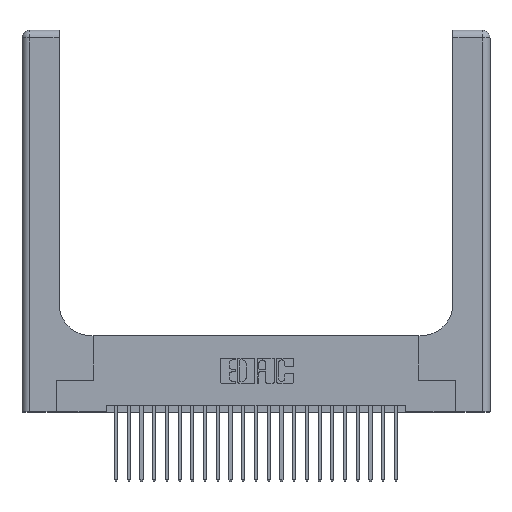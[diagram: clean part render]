
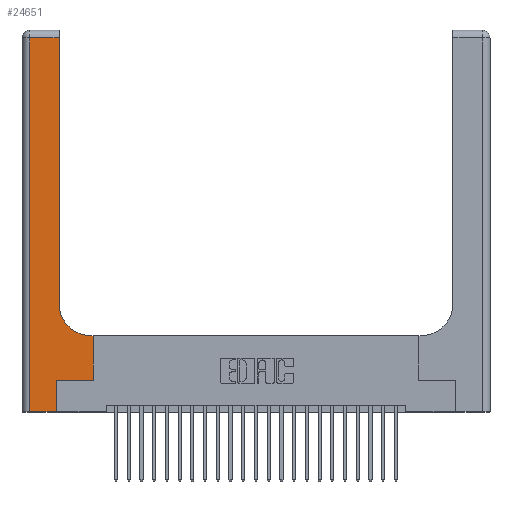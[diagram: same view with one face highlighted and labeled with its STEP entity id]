
A CAD part, top view. The second image highlights one B-rep face of the part: STEP entity #24651.
In plain terms, the highlighted planar face has unit normal (0, 0, 1).
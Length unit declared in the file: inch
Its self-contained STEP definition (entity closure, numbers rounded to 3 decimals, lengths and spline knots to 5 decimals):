
#49 = CARTESIAN_POINT ( 'NONE',  ( 0., 2.94, 0.37 ) ) ;
#274 = CARTESIAN_POINT ( 'NONE',  ( 0.5585, 0.6, 0.37 ) ) ;
#1106 = CARTESIAN_POINT ( 'NONE',  ( 0.5585, 0.25, 0.37 ) ) ;
#1287 = EDGE_CURVE ( 'NONE', #21738, #24927, #8730, .T. ) ;
#1497 = ORIENTED_EDGE ( 'NONE', *, *, #2717, .T. ) ;
#1663 = CARTESIAN_POINT ( 'NONE',  ( 0.2915, 3., 0.37 ) ) ;
#1763 = CARTESIAN_POINT ( 'NONE',  ( 0.5585, 0.25, 0.37 ) ) ;
#1815 = ORIENTED_EDGE ( 'NONE', *, *, #3373, .T. ) ;
#2321 = VERTEX_POINT ( 'NONE', #20950 ) ;
#2422 = LINE ( 'NONE', #19291, #16740 ) ;
#2436 = EDGE_CURVE ( 'NONE', #24927, #21970, #2422, .T. ) ;
#2717 = EDGE_CURVE ( 'NONE', #21970, #18463, #4589, .T. ) ;
#2721 = VECTOR ( 'NONE', #18853, 39.37008 ) ;
#3373 = EDGE_CURVE ( 'NONE', #8254, #21738, #21654, .T. ) ;
#3659 = DIRECTION ( 'NONE',  ( 0., 1., 0. ) ) ;
#4030 = DIRECTION ( 'NONE',  ( 0., 1., 0. ) ) ;
#4109 = EDGE_CURVE ( 'NONE', #18463, #8158, #24777, .T. ) ;
#4205 = ORIENTED_EDGE ( 'NONE', *, *, #1287, .T. ) ;
#4511 = CARTESIAN_POINT ( 'NONE',  ( 0.269, 0.25, 0.37 ) ) ;
#4589 = LINE ( 'NONE', #20913, #2721 ) ;
#4878 = CIRCLE ( 'NONE', #7645, 0.25 ) ;
#5164 = ORIENTED_EDGE ( 'NONE', *, *, #12027, .T. ) ;
#5552 = DIRECTION ( 'NONE',  ( 1., 0., 0. ) ) ;
#5937 = EDGE_CURVE ( 'NONE', #2321, #8254, #16563, .T. ) ;
#6708 = CARTESIAN_POINT ( 'NONE',  ( 0.2915, 0.6, 0.37 ) ) ;
#6750 = VECTOR ( 'NONE', #15170, 39.37008 ) ;
#6876 = ORIENTED_EDGE ( 'NONE', *, *, #24856, .T. ) ;
#6952 = DIRECTION ( 'NONE',  ( 0., 0., -1. ) ) ;
#7208 = CARTESIAN_POINT ( 'NONE',  ( 0.269, 0., 0.37 ) ) ;
#7543 = VECTOR ( 'NONE', #18272, 39.37008 ) ;
#7645 = AXIS2_PLACEMENT_3D ( 'NONE', #17139, #6952, #22876 ) ;
#7898 = LINE ( 'NONE', #6708, #23797 ) ;
#8158 = VERTEX_POINT ( 'NONE', #274 ) ;
#8254 = VERTEX_POINT ( 'NONE', #23902 ) ;
#8629 = DIRECTION ( 'NONE',  ( -1., 0., 0. ) ) ;
#8708 = CARTESIAN_POINT ( 'NONE',  ( 0.5415, 0.6, 0.37 ) ) ;
#8730 = LINE ( 'NONE', #21828, #9941 ) ;
#9941 = VECTOR ( 'NONE', #5552, 39.37008 ) ;
#11028 = VECTOR ( 'NONE', #23143, 39.37008 ) ;
#11430 = AXIS2_PLACEMENT_3D ( 'NONE', #24208, #23947, #12202 ) ;
#12027 = EDGE_CURVE ( 'NONE', #21786, #2321, #12137, .T. ) ;
#12031 = ORIENTED_EDGE ( 'NONE', *, *, #2436, .T. ) ;
#12137 = LINE ( 'NONE', #1663, #18773 ) ;
#12202 = DIRECTION ( 'NONE',  ( -1., 0., 0. ) ) ;
#13528 = CARTESIAN_POINT ( 'NONE',  ( 0.2915, 0.85, 0.37 ) ) ;
#15170 = DIRECTION ( 'NONE',  ( 0., -1., 0. ) ) ;
#15350 = VERTEX_POINT ( 'NONE', #8708 ) ;
#15661 = PLANE ( 'NONE',  #11430 ) ;
#16521 = EDGE_LOOP ( 'NONE', ( #5164, #25117, #1815, #4205, #12031, #1497, #24893, #17490, #6876 ) ) ;
#16563 = LINE ( 'NONE', #49, #7543 ) ;
#16740 = VECTOR ( 'NONE', #4030, 39.37008 ) ;
#17139 = CARTESIAN_POINT ( 'NONE',  ( 0.5415, 0.85, 0.37 ) ) ;
#17366 = FACE_OUTER_BOUND ( 'NONE', #16521, .T. ) ;
#17490 = ORIENTED_EDGE ( 'NONE', *, *, #18688, .T. ) ;
#18272 = DIRECTION ( 'NONE',  ( -1., 0., 0. ) ) ;
#18463 = VERTEX_POINT ( 'NONE', #1763 ) ;
#18688 = EDGE_CURVE ( 'NONE', #8158, #15350, #7898, .T. ) ;
#18773 = VECTOR ( 'NONE', #3659, 39.37008 ) ;
#18853 = DIRECTION ( 'NONE',  ( 1., 0., 0. ) ) ;
#19291 = CARTESIAN_POINT ( 'NONE',  ( 0.269, 0., 0.37 ) ) ;
#19365 = CARTESIAN_POINT ( 'NONE',  ( 0.06, 3., 0.37 ) ) ;
#20913 = CARTESIAN_POINT ( 'NONE',  ( 0.269, 0.25, 0.37 ) ) ;
#20950 = CARTESIAN_POINT ( 'NONE',  ( 0.2915, 2.94, 0.37 ) ) ;
#21654 = LINE ( 'NONE', #19365, #6750 ) ;
#21738 = VERTEX_POINT ( 'NONE', #25527 ) ;
#21786 = VERTEX_POINT ( 'NONE', #13528 ) ;
#21828 = CARTESIAN_POINT ( 'NONE',  ( 0., 0., 0.37 ) ) ;
#21970 = VERTEX_POINT ( 'NONE', #4511 ) ;
#22876 = DIRECTION ( 'NONE',  ( 1., 0., 0. ) ) ;
#23143 = DIRECTION ( 'NONE',  ( 0., 1., 0. ) ) ;
#23797 = VECTOR ( 'NONE', #8629, 39.37008 ) ;
#23902 = CARTESIAN_POINT ( 'NONE',  ( 0.06, 2.94, 0.37 ) ) ;
#23947 = DIRECTION ( 'NONE',  ( 0., 0., -1. ) ) ;
#24208 = CARTESIAN_POINT ( 'NONE',  ( 0., 3., 0.37 ) ) ;
#24651 = ADVANCED_FACE ( 'NONE', ( #17366 ), #15661, .F. ) ;
#24777 = LINE ( 'NONE', #1106, #11028 ) ;
#24856 = EDGE_CURVE ( 'NONE', #15350, #21786, #4878, .T. ) ;
#24893 = ORIENTED_EDGE ( 'NONE', *, *, #4109, .T. ) ;
#24927 = VERTEX_POINT ( 'NONE', #7208 ) ;
#25117 = ORIENTED_EDGE ( 'NONE', *, *, #5937, .T. ) ;
#25527 = CARTESIAN_POINT ( 'NONE',  ( 0.06, 0., 0.37 ) ) ;
